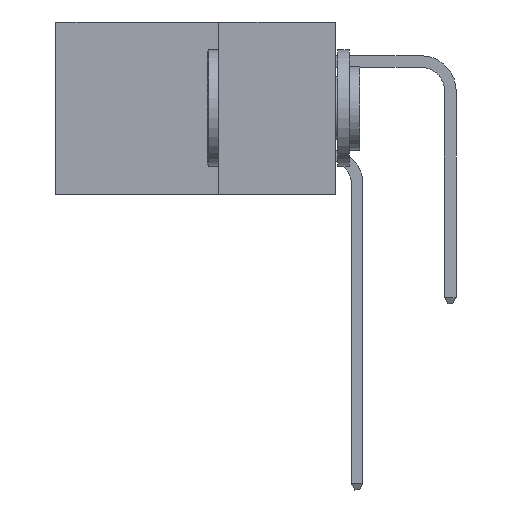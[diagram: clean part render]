
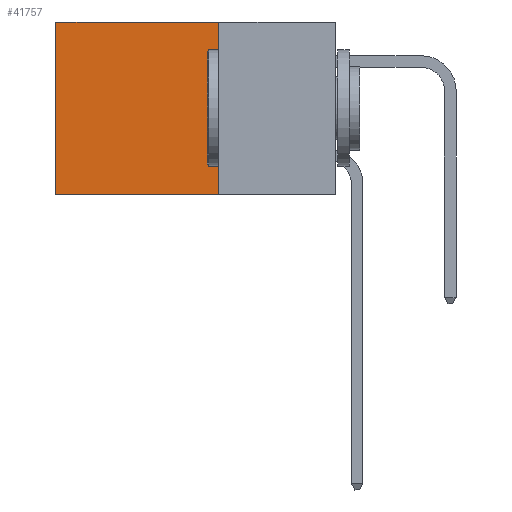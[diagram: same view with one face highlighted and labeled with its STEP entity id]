
A CAD part, left-side view. The second image highlights one B-rep face of the part: STEP entity #41757.
In plain terms, the highlighted planar face has unit normal (-1, 0, 0).
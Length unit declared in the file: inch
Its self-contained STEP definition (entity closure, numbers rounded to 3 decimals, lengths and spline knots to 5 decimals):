
#408 = EDGE_CURVE ( 'NONE', #10711, #34261, #29581, .T. ) ;
#3530 = ORIENTED_EDGE ( 'NONE', *, *, #408, .T. ) ;
#5054 = EDGE_CURVE ( 'NONE', #10711, #6209, #19855, .T. ) ;
#5229 = VECTOR ( 'NONE', #39771, 39.37008 ) ;
#5268 = DIRECTION ( 'NONE',  ( 0., 0., -1. ) ) ;
#6209 = VERTEX_POINT ( 'NONE', #33798 ) ;
#6672 = CARTESIAN_POINT ( 'NONE',  ( 0.2875, 0.25, -0.37 ) ) ;
#7965 = EDGE_LOOP ( 'NONE', ( #22278, #44484, #36217, #3530 ) ) ;
#8686 = CARTESIAN_POINT ( 'NONE',  ( 0.2875, 0.6, -0.37 ) ) ;
#9462 = VECTOR ( 'NONE', #37549, 39.37008 ) ;
#10711 = VERTEX_POINT ( 'NONE', #37240 ) ;
#14309 = VECTOR ( 'NONE', #38053, 39.37008 ) ;
#16628 = CARTESIAN_POINT ( 'NONE',  ( 0.2875, 0.25, 0. ) ) ;
#18412 = LINE ( 'NONE', #6672, #9462 ) ;
#19855 = LINE ( 'NONE', #16628, #14309 ) ;
#22278 = ORIENTED_EDGE ( 'NONE', *, *, #33349, .T. ) ;
#22801 = FACE_OUTER_BOUND ( 'NONE', #7965, .T. ) ;
#23081 = VERTEX_POINT ( 'NONE', #8686 ) ;
#26465 = PLANE ( 'NONE',  #35727 ) ;
#27422 = CARTESIAN_POINT ( 'NONE',  ( 0.2875, 0.6, 0. ) ) ;
#29512 = LINE ( 'NONE', #40722, #41017 ) ;
#29581 = LINE ( 'NONE', #34430, #5229 ) ;
#29857 = DIRECTION ( 'NONE',  ( 1., 0., 0. ) ) ;
#29974 = DIRECTION ( 'NONE',  ( 0., 0., -1. ) ) ;
#33349 = EDGE_CURVE ( 'NONE', #34261, #23081, #29512, .T. ) ;
#33680 = CARTESIAN_POINT ( 'NONE',  ( 0.2875, 0.25, 0. ) ) ;
#33798 = CARTESIAN_POINT ( 'NONE',  ( 0.2875, 0.25, -0.37 ) ) ;
#34261 = VERTEX_POINT ( 'NONE', #27422 ) ;
#34430 = CARTESIAN_POINT ( 'NONE',  ( 0.2875, 0.25, 0. ) ) ;
#35727 = AXIS2_PLACEMENT_3D ( 'NONE', #33680, #29857, #5268 ) ;
#36217 = ORIENTED_EDGE ( 'NONE', *, *, #5054, .F. ) ;
#37240 = CARTESIAN_POINT ( 'NONE',  ( 0.2875, 0.25, 0. ) ) ;
#37549 = DIRECTION ( 'NONE',  ( 0., 1., 0. ) ) ;
#38053 = DIRECTION ( 'NONE',  ( 0., 0., -1. ) ) ;
#39771 = DIRECTION ( 'NONE',  ( 0., 1., 0. ) ) ;
#40722 = CARTESIAN_POINT ( 'NONE',  ( 0.2875, 0.6, 0. ) ) ;
#41017 = VECTOR ( 'NONE', #29974, 39.37008 ) ;
#41255 = EDGE_CURVE ( 'NONE', #6209, #23081, #18412, .T. ) ;
#41757 = ADVANCED_FACE ( 'NONE', ( #22801 ), #26465, .F. ) ;
#44484 = ORIENTED_EDGE ( 'NONE', *, *, #41255, .F. ) ;
